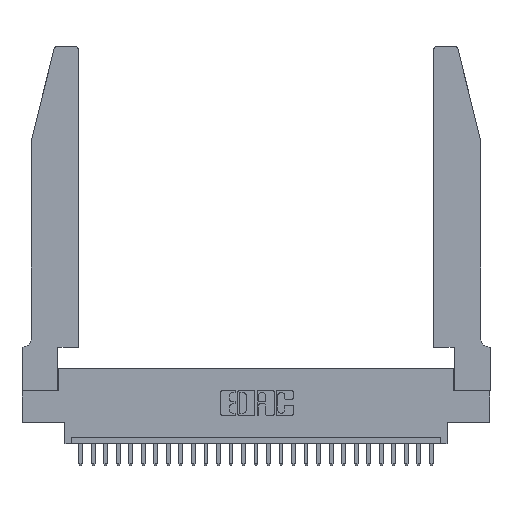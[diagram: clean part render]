
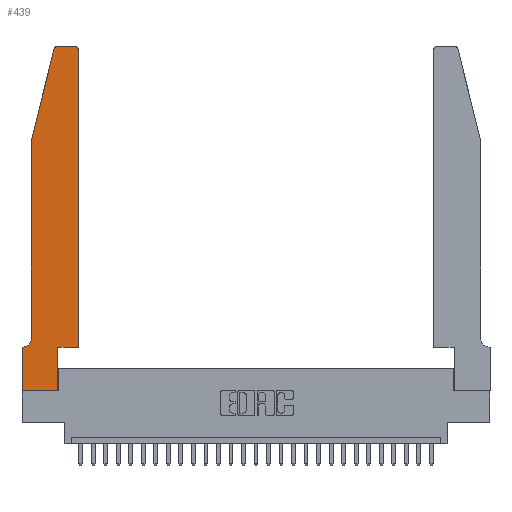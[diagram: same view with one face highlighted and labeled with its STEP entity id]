
A CAD part, top view. The second image highlights one B-rep face of the part: STEP entity #439.
In plain terms, the highlighted planar face has unit normal (0, 0, 1).
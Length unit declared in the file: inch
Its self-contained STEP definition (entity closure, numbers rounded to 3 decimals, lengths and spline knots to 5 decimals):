
#439 = ADVANCED_FACE ( 'NONE', ( #18760 ), #7873, .T. ) ;
#571 = CARTESIAN_POINT ( 'NONE',  ( 0.4505, 0.35, 0.37 ) ) ;
#1315 = VERTEX_POINT ( 'NONE', #28419 ) ;
#1325 = CIRCLE ( 'NONE', #19912, 0.07 ) ;
#1426 = CARTESIAN_POINT ( 'NONE',  ( 0.2865, 0.35, 0.37 ) ) ;
#1606 = CARTESIAN_POINT ( 'NONE',  ( 0.2865, 0.35, 0.37 ) ) ;
#1990 = LINE ( 'NONE', #14981, #8510 ) ;
#2111 = VERTEX_POINT ( 'NONE', #21238 ) ;
#2328 = CARTESIAN_POINT ( 'NONE',  ( 0.284, 2.72, 0.37 ) ) ;
#2368 = VERTEX_POINT ( 'NONE', #18341 ) ;
#2587 = LINE ( 'NONE', #20656, #5682 ) ;
#2790 = CARTESIAN_POINT ( 'NONE',  ( 0.0755, 2., 0.37 ) ) ;
#3020 = AXIS2_PLACEMENT_3D ( 'NONE', #2328, #24276, #26324 ) ;
#3048 = ORIENTED_EDGE ( 'NONE', *, *, #27655, .T. ) ;
#3454 = VECTOR ( 'NONE', #20401, 39.37008 ) ;
#4175 = CIRCLE ( 'NONE', #3020, 0.03 ) ;
#4744 = VERTEX_POINT ( 'NONE', #26236 ) ;
#5014 = CARTESIAN_POINT ( 'NONE',  ( 0., 0., 0.37 ) ) ;
#5590 = ORIENTED_EDGE ( 'NONE', *, *, #18131, .T. ) ;
#5682 = VECTOR ( 'NONE', #20363, 39.37008 ) ;
#5940 = VERTEX_POINT ( 'NONE', #5014 ) ;
#6463 = EDGE_CURVE ( 'NONE', #24518, #2368, #27900, .T. ) ;
#6620 = CIRCLE ( 'NONE', #26369, 0.03 ) ;
#6623 = VERTEX_POINT ( 'NONE', #1426 ) ;
#6877 = VERTEX_POINT ( 'NONE', #16294 ) ;
#6997 = VECTOR ( 'NONE', #17645, 39.37008 ) ;
#7184 = CARTESIAN_POINT ( 'NONE',  ( 0.25487, 2.72718, 0.37 ) ) ;
#7843 = AXIS2_PLACEMENT_3D ( 'NONE', #28200, #18403, #9276 ) ;
#7873 = PLANE ( 'NONE',  #7843 ) ;
#8365 = VECTOR ( 'NONE', #25839, 39.37008 ) ;
#8510 = VECTOR ( 'NONE', #12866, 39.37008 ) ;
#8557 = VECTOR ( 'NONE', #17311, 39.37008 ) ;
#8634 = EDGE_CURVE ( 'NONE', #14217, #17778, #6620, .T. ) ;
#8713 = CARTESIAN_POINT ( 'NONE',  ( 0.4505, 0.35, 0.37 ) ) ;
#8809 = ORIENTED_EDGE ( 'NONE', *, *, #8634, .T. ) ;
#9276 = DIRECTION ( 'NONE',  ( 1., 0., 0. ) ) ;
#9644 = DIRECTION ( 'NONE',  ( 0., 0., -1. ) ) ;
#9682 = ORIENTED_EDGE ( 'NONE', *, *, #13514, .T. ) ;
#10212 = VECTOR ( 'NONE', #18814, 39.37008 ) ;
#11626 = CARTESIAN_POINT ( 'NONE',  ( 0.4205, 2.75, 0.37 ) ) ;
#11644 = VECTOR ( 'NONE', #18059, 39.37008 ) ;
#11975 = CARTESIAN_POINT ( 'NONE',  ( 0.4205, 2.72, 0.37 ) ) ;
#12028 = EDGE_CURVE ( 'NONE', #5940, #15942, #18275, .T. ) ;
#12376 = EDGE_CURVE ( 'NONE', #1315, #4744, #1325, .T. ) ;
#12693 = ORIENTED_EDGE ( 'NONE', *, *, #6463, .T. ) ;
#12866 = DIRECTION ( 'NONE',  ( -1., 0., 0. ) ) ;
#13205 = ORIENTED_EDGE ( 'NONE', *, *, #14753, .T. ) ;
#13514 = EDGE_CURVE ( 'NONE', #15942, #6623, #26283, .T. ) ;
#13914 = CARTESIAN_POINT ( 'NONE',  ( 0.0055, 0.42, 0.37 ) ) ;
#14217 = VERTEX_POINT ( 'NONE', #16847 ) ;
#14343 = CARTESIAN_POINT ( 'NONE',  ( 0.2865, 0., 0.37 ) ) ;
#14512 = VERTEX_POINT ( 'NONE', #571 ) ;
#14649 = ORIENTED_EDGE ( 'NONE', *, *, #12028, .T. ) ;
#14753 = EDGE_CURVE ( 'NONE', #17778, #6877, #1990, .T. ) ;
#14981 = CARTESIAN_POINT ( 'NONE',  ( 0.2605, 2.75, 0.37 ) ) ;
#15107 = EDGE_CURVE ( 'NONE', #14512, #14217, #26491, .T. ) ;
#15942 = VERTEX_POINT ( 'NONE', #14343 ) ;
#16294 = CARTESIAN_POINT ( 'NONE',  ( 0.284, 2.75, 0.37 ) ) ;
#16390 = DIRECTION ( 'NONE',  ( 1., 0., 0. ) ) ;
#16559 = EDGE_CURVE ( 'NONE', #4744, #2111, #20158, .T. ) ;
#16692 = CARTESIAN_POINT ( 'NONE',  ( 0.4505, 0.35, 0.37 ) ) ;
#16847 = CARTESIAN_POINT ( 'NONE',  ( 0.4505, 2.72, 0.37 ) ) ;
#17041 = DIRECTION ( 'NONE',  ( 0., 1., 0. ) ) ;
#17311 = DIRECTION ( 'NONE',  ( 1., 0., 0. ) ) ;
#17645 = DIRECTION ( 'NONE',  ( 1., 0., 0. ) ) ;
#17778 = VERTEX_POINT ( 'NONE', #11626 ) ;
#18059 = DIRECTION ( 'NONE',  ( -0.239, -0.971, 0. ) ) ;
#18131 = EDGE_CURVE ( 'NONE', #2368, #1315, #20443, .T. ) ;
#18275 = LINE ( 'NONE', #27867, #8557 ) ;
#18341 = CARTESIAN_POINT ( 'NONE',  ( 0.0755, 2., 0.37 ) ) ;
#18403 = DIRECTION ( 'NONE',  ( 0., 0., 1. ) ) ;
#18760 = FACE_OUTER_BOUND ( 'NONE', #28125, .T. ) ;
#18814 = DIRECTION ( 'NONE',  ( 0., 1., 0. ) ) ;
#18997 = VECTOR ( 'NONE', #17041, 39.37008 ) ;
#19789 = ORIENTED_EDGE ( 'NONE', *, *, #15107, .T. ) ;
#19912 = AXIS2_PLACEMENT_3D ( 'NONE', #13914, #9644, #25138 ) ;
#20002 = EDGE_CURVE ( 'NONE', #2111, #5940, #2587, .T. ) ;
#20158 = LINE ( 'NONE', #25344, #8365 ) ;
#20306 = CARTESIAN_POINT ( 'NONE',  ( 0.0755, 2., 0.37 ) ) ;
#20363 = DIRECTION ( 'NONE',  ( 0., -1., 0. ) ) ;
#20401 = DIRECTION ( 'NONE',  ( 0., -1., 0. ) ) ;
#20432 = ORIENTED_EDGE ( 'NONE', *, *, #12376, .T. ) ;
#20443 = LINE ( 'NONE', #20306, #3454 ) ;
#20541 = ORIENTED_EDGE ( 'NONE', *, *, #25625, .T. ) ;
#20656 = CARTESIAN_POINT ( 'NONE',  ( 0., 0., 0.37 ) ) ;
#21238 = CARTESIAN_POINT ( 'NONE',  ( 0., 0.35, 0.37 ) ) ;
#24276 = DIRECTION ( 'NONE',  ( 0., 0., 1. ) ) ;
#24286 = ORIENTED_EDGE ( 'NONE', *, *, #16559, .T. ) ;
#24518 = VERTEX_POINT ( 'NONE', #7184 ) ;
#25138 = DIRECTION ( 'NONE',  ( -1., 0., 0. ) ) ;
#25344 = CARTESIAN_POINT ( 'NONE',  ( 0.0755, 0.35, 0.37 ) ) ;
#25625 = EDGE_CURVE ( 'NONE', #6623, #14512, #28180, .T. ) ;
#25839 = DIRECTION ( 'NONE',  ( -1., 0., 0. ) ) ;
#26236 = CARTESIAN_POINT ( 'NONE',  ( 0.0055, 0.35, 0.37 ) ) ;
#26283 = LINE ( 'NONE', #1606, #18997 ) ;
#26324 = DIRECTION ( 'NONE',  ( 1., 0., 0. ) ) ;
#26369 = AXIS2_PLACEMENT_3D ( 'NONE', #11975, #27424, #16390 ) ;
#26491 = LINE ( 'NONE', #16692, #10212 ) ;
#27424 = DIRECTION ( 'NONE',  ( 0., 0., 1. ) ) ;
#27655 = EDGE_CURVE ( 'NONE', #6877, #24518, #4175, .T. ) ;
#27867 = CARTESIAN_POINT ( 'NONE',  ( 0., 0., 0.37 ) ) ;
#27900 = LINE ( 'NONE', #2790, #11644 ) ;
#27971 = ORIENTED_EDGE ( 'NONE', *, *, #20002, .T. ) ;
#28125 = EDGE_LOOP ( 'NONE', ( #13205, #3048, #12693, #5590, #20432, #24286, #27971, #14649, #9682, #20541, #19789, #8809 ) ) ;
#28180 = LINE ( 'NONE', #8713, #6997 ) ;
#28200 = CARTESIAN_POINT ( 'NONE',  ( 0., 0.35, 0.37 ) ) ;
#28419 = CARTESIAN_POINT ( 'NONE',  ( 0.0755, 0.42, 0.37 ) ) ;
